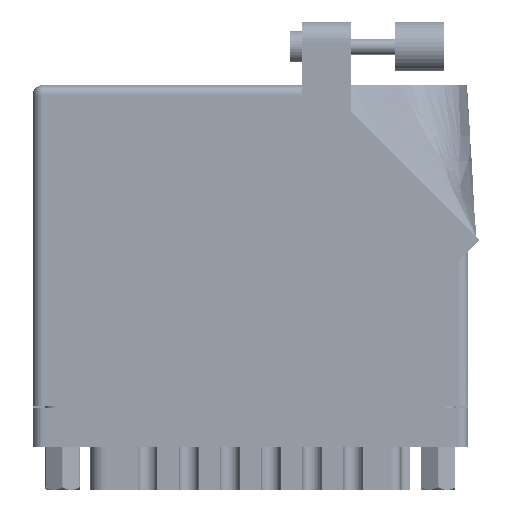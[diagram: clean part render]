
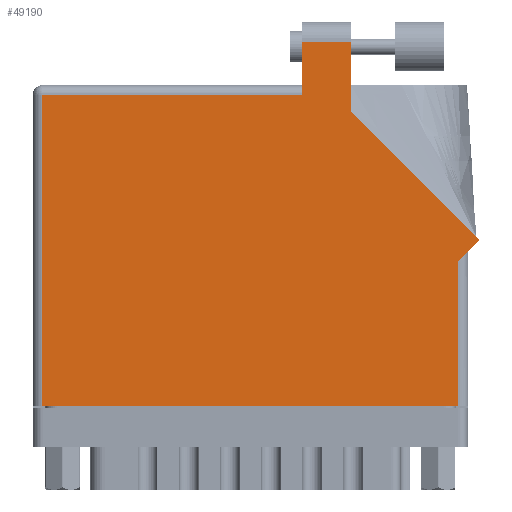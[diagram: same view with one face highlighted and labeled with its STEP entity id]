
A CAD part, front view. The second image highlights one B-rep face of the part: STEP entity #49190.
In plain terms, the highlighted face is planar.
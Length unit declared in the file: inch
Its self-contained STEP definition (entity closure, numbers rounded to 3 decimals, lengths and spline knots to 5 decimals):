
#45 = CARTESIAN_POINT ( 'NONE',  ( 0.062, 0., 0. ) ) ;
#541 = CARTESIAN_POINT ( 'NONE',  ( 0., 2.03, 0. ) ) ;
#2599 = VECTOR ( 'NONE', #49149, 39.37008 ) ;
#2817 = LINE ( 'NONE', #94055, #71340 ) ;
#2906 = LINE ( 'NONE', #102203, #15058 ) ;
#4504 = VERTEX_POINT ( 'NONE', #65486 ) ;
#5577 = CARTESIAN_POINT ( 'NONE',  ( 2.693, 0.98, 0. ) ) ;
#8487 = CARTESIAN_POINT ( 'NONE',  ( 0., 1.968, 0. ) ) ;
#8997 = ORIENTED_EDGE ( 'NONE', *, *, #82070, .T. ) ;
#9597 = ORIENTED_EDGE ( 'NONE', *, *, #32094, .T. ) ;
#10181 = PLANE ( 'NONE',  #23818 ) ;
#10809 = ORIENTED_EDGE ( 'NONE', *, *, #38404, .T. ) ;
#10897 = DIRECTION ( 'NONE',  ( -1., 0., 0. ) ) ;
#11024 = VECTOR ( 'NONE', #57413, 39.37008 ) ;
#11953 = LINE ( 'NONE', #84418, #103002 ) ;
#13524 = EDGE_CURVE ( 'NONE', #44288, #24228, #65801, .T. ) ;
#15017 = EDGE_CURVE ( 'NONE', #4504, #67007, #2817, .T. ) ;
#15058 = VECTOR ( 'NONE', #84500, 39.37008 ) ;
#16528 = CARTESIAN_POINT ( 'NONE',  ( 2.693, 0.918, 0. ) ) ;
#17567 = CARTESIAN_POINT ( 'NONE',  ( 2.82571, 1.05071, 0. ) ) ;
#17572 = LINE ( 'NONE', #18091, #74586 ) ;
#18091 = CARTESIAN_POINT ( 'NONE',  ( 2.012, 1.86442, 0. ) ) ;
#21988 = VERTEX_POINT ( 'NONE', #16528 ) ;
#23818 = AXIS2_PLACEMENT_3D ( 'NONE', #541, #66038, #42401 ) ;
#24168 = ORIENTED_EDGE ( 'NONE', *, *, #13524, .T. ) ;
#24228 = VERTEX_POINT ( 'NONE', #78861 ) ;
#30293 = DIRECTION ( 'NONE',  ( 0., 1., 0. ) ) ;
#32094 = EDGE_CURVE ( 'NONE', #71125, #91230, #11953, .T. ) ;
#32821 = DIRECTION ( 'NONE',  ( 0., -1., 0. ) ) ;
#33779 = CARTESIAN_POINT ( 'NONE',  ( 1.705, 2.03, 0. ) ) ;
#34315 = LINE ( 'NONE', #33779, #11024 ) ;
#35261 = VERTEX_POINT ( 'NONE', #50112 ) ;
#38404 = EDGE_CURVE ( 'NONE', #24228, #71125, #17572, .T. ) ;
#40353 = CARTESIAN_POINT ( 'NONE',  ( 1.705, 1.968, 0. ) ) ;
#41247 = DIRECTION ( 'NONE',  ( -1., 0., 0. ) ) ;
#41834 = VECTOR ( 'NONE', #32821, 39.37008 ) ;
#42401 = DIRECTION ( 'NONE',  ( -1., 0., 0. ) ) ;
#44288 = VERTEX_POINT ( 'NONE', #17567 ) ;
#46213 = EDGE_CURVE ( 'NONE', #21988, #44288, #2906, .T. ) ;
#48853 = FACE_OUTER_BOUND ( 'NONE', #74920, .T. ) ;
#49149 = DIRECTION ( 'NONE',  ( -0.707, 0.707, 0. ) ) ;
#49190 = ADVANCED_FACE ( 'NONE', ( #48853 ), #10181, .F. ) ;
#50112 = CARTESIAN_POINT ( 'NONE',  ( 0.062, 1.968, 0. ) ) ;
#51578 = ORIENTED_EDGE ( 'NONE', *, *, #46213, .T. ) ;
#52192 = ORIENTED_EDGE ( 'NONE', *, *, #92878, .T. ) ;
#55485 = VERTEX_POINT ( 'NONE', #40353 ) ;
#57413 = DIRECTION ( 'NONE',  ( 0., -1., 0. ) ) ;
#58314 = ORIENTED_EDGE ( 'NONE', *, *, #15017, .T. ) ;
#59023 = CARTESIAN_POINT ( 'NONE',  ( 2.012, 2.305, 0. ) ) ;
#59202 = ORIENTED_EDGE ( 'NONE', *, *, #82591, .T. ) ;
#60619 = VECTOR ( 'NONE', #30293, 39.37008 ) ;
#64328 = EDGE_CURVE ( 'NONE', #91230, #55485, #34315, .T. ) ;
#65486 = CARTESIAN_POINT ( 'NONE',  ( 0.062, 0., 0. ) ) ;
#65801 = LINE ( 'NONE', #98525, #2599 ) ;
#66038 = DIRECTION ( 'NONE',  ( 0., 0., -1. ) ) ;
#67007 = VERTEX_POINT ( 'NONE', #86333 ) ;
#71125 = VERTEX_POINT ( 'NONE', #59023 ) ;
#71340 = VECTOR ( 'NONE', #78452, 39.37008 ) ;
#73607 = LINE ( 'NONE', #45, #41834 ) ;
#74586 = VECTOR ( 'NONE', #90547, 39.37008 ) ;
#74920 = EDGE_LOOP ( 'NONE', ( #10809, #9597, #100947, #52192, #59202, #58314, #8997, #51578, #24168 ) ) ;
#78452 = DIRECTION ( 'NONE',  ( 1., 0., 0. ) ) ;
#78861 = CARTESIAN_POINT ( 'NONE',  ( 2.012, 1.86442, 0. ) ) ;
#79116 = LINE ( 'NONE', #5577, #60619 ) ;
#81786 = CARTESIAN_POINT ( 'NONE',  ( 1.705, 2.305, 0. ) ) ;
#82021 = LINE ( 'NONE', #8487, #105699 ) ;
#82070 = EDGE_CURVE ( 'NONE', #67007, #21988, #79116, .T. ) ;
#82591 = EDGE_CURVE ( 'NONE', #35261, #4504, #73607, .T. ) ;
#84418 = CARTESIAN_POINT ( 'NONE',  ( 1.705, 2.305, 0. ) ) ;
#84500 = DIRECTION ( 'NONE',  ( 0.707, 0.707, 0. ) ) ;
#86333 = CARTESIAN_POINT ( 'NONE',  ( 2.693, 0., 0. ) ) ;
#90547 = DIRECTION ( 'NONE',  ( 0., 1., 0. ) ) ;
#91230 = VERTEX_POINT ( 'NONE', #81786 ) ;
#92878 = EDGE_CURVE ( 'NONE', #55485, #35261, #82021, .T. ) ;
#94055 = CARTESIAN_POINT ( 'NONE',  ( 0., 0., 0. ) ) ;
#98525 = CARTESIAN_POINT ( 'NONE',  ( 2.82571, 1.05071, 0. ) ) ;
#100947 = ORIENTED_EDGE ( 'NONE', *, *, #64328, .T. ) ;
#102203 = CARTESIAN_POINT ( 'NONE',  ( 2.755, 0.98, 0. ) ) ;
#103002 = VECTOR ( 'NONE', #10897, 39.37008 ) ;
#105699 = VECTOR ( 'NONE', #41247, 39.37008 ) ;
